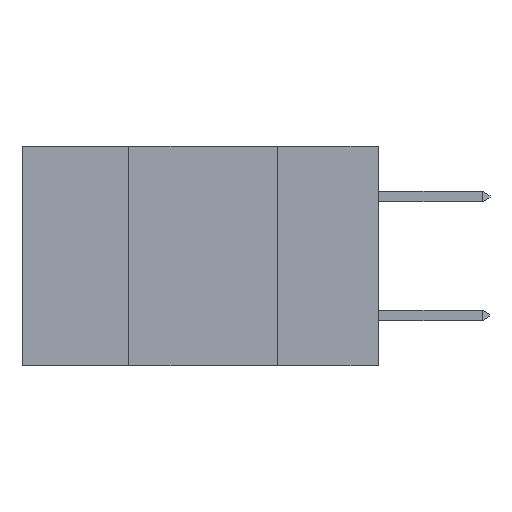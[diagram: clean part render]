
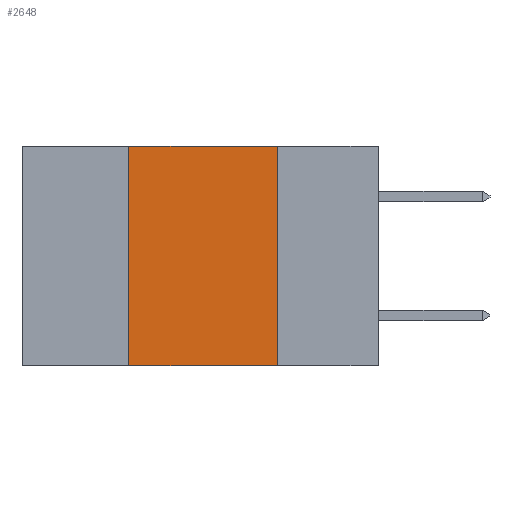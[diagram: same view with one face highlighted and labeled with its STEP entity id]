
A CAD part, left-side view. The second image highlights one B-rep face of the part: STEP entity #2648.
In plain terms, the highlighted planar face has unit normal (-1, 0, 0).
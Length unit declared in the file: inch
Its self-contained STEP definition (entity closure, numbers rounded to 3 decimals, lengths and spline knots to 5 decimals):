
#23 = VERTEX_POINT ( 'NONE', #1252 ) ;
#102 = LINE ( 'NONE', #2865, #3319 ) ;
#659 = FACE_OUTER_BOUND ( 'NONE', #4708, .T. ) ;
#1093 = EDGE_CURVE ( 'NONE', #6813, #23, #4140, .T. ) ;
#1225 = VERTEX_POINT ( 'NONE', #13008 ) ;
#1252 = CARTESIAN_POINT ( 'NONE',  ( 0., 0.42, 0. ) ) ;
#1472 = CARTESIAN_POINT ( 'NONE',  ( 0., 0.42, -0.37 ) ) ;
#1502 = EDGE_CURVE ( 'NONE', #23, #1225, #2488, .T. ) ;
#2488 = LINE ( 'NONE', #6241, #10602 ) ;
#2648 = ADVANCED_FACE ( 'NONE', ( #659 ), #10246, .F. ) ;
#2828 = DIRECTION ( 'NONE',  ( 0., -1., 0. ) ) ;
#2865 = CARTESIAN_POINT ( 'NONE',  ( 0., 0.6, -0.37 ) ) ;
#3121 = VERTEX_POINT ( 'NONE', #13084 ) ;
#3177 = DIRECTION ( 'NONE',  ( 0., 0., -1. ) ) ;
#3319 = VECTOR ( 'NONE', #2828, 39.37008 ) ;
#3511 = DIRECTION ( 'NONE',  ( 0., 0., 1. ) ) ;
#4140 = LINE ( 'NONE', #8706, #12054 ) ;
#4209 = ORIENTED_EDGE ( 'NONE', *, *, #4735, .F. ) ;
#4392 = ORIENTED_EDGE ( 'NONE', *, *, #1502, .F. ) ;
#4708 = EDGE_LOOP ( 'NONE', ( #4209, #4392, #5093, #5610 ) ) ;
#4718 = AXIS2_PLACEMENT_3D ( 'NONE', #12058, #9653, #3177 ) ;
#4735 = EDGE_CURVE ( 'NONE', #1225, #3121, #11907, .T. ) ;
#4906 = DIRECTION ( 'NONE',  ( 0., -1., 0. ) ) ;
#5093 = ORIENTED_EDGE ( 'NONE', *, *, #1093, .F. ) ;
#5610 = ORIENTED_EDGE ( 'NONE', *, *, #8744, .T. ) ;
#6241 = CARTESIAN_POINT ( 'NONE',  ( 0., 0.6, 0. ) ) ;
#6779 = CARTESIAN_POINT ( 'NONE',  ( 0., 0.17, 0. ) ) ;
#6813 = VERTEX_POINT ( 'NONE', #1472 ) ;
#7274 = DIRECTION ( 'NONE',  ( 0., 0., -1. ) ) ;
#8706 = CARTESIAN_POINT ( 'NONE',  ( 0., 0.42, 0. ) ) ;
#8744 = EDGE_CURVE ( 'NONE', #6813, #3121, #102, .T. ) ;
#9224 = VECTOR ( 'NONE', #7274, 39.37008 ) ;
#9653 = DIRECTION ( 'NONE',  ( 1., 0., 0. ) ) ;
#10246 = PLANE ( 'NONE',  #4718 ) ;
#10602 = VECTOR ( 'NONE', #4906, 39.37008 ) ;
#11907 = LINE ( 'NONE', #6779, #9224 ) ;
#12054 = VECTOR ( 'NONE', #3511, 39.37008 ) ;
#12058 = CARTESIAN_POINT ( 'NONE',  ( 0., 0.6, 0. ) ) ;
#13008 = CARTESIAN_POINT ( 'NONE',  ( 0., 0.17, 0. ) ) ;
#13084 = CARTESIAN_POINT ( 'NONE',  ( 0., 0.17, -0.37 ) ) ;
